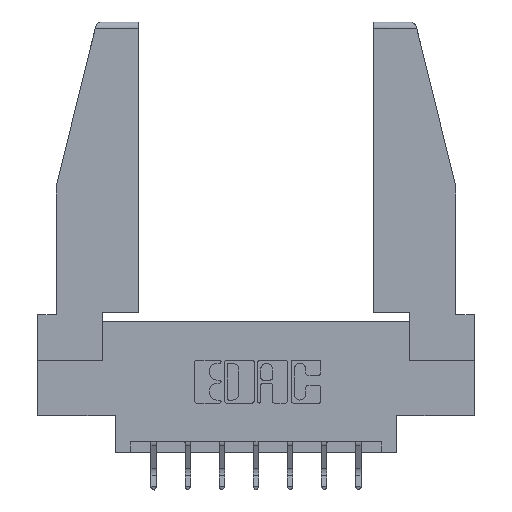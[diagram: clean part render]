
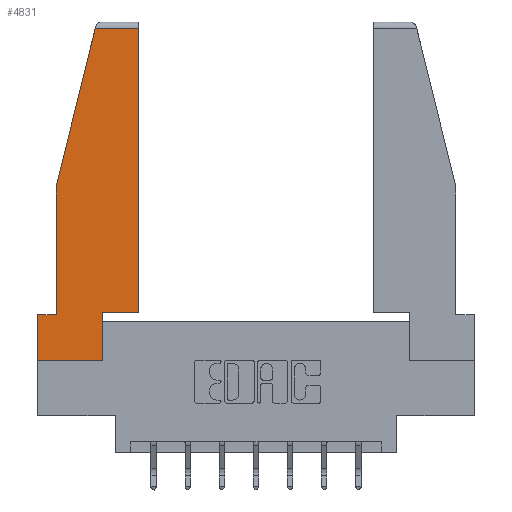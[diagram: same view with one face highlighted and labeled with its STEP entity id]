
A CAD part, top view. The second image highlights one B-rep face of the part: STEP entity #4831.
In plain terms, the highlighted planar face has unit normal (0, 0, 1).
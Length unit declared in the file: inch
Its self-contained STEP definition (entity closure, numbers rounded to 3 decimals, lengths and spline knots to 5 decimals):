
#357 = DIRECTION ( 'NONE',  ( 1., 0., 0. ) ) ;
#682 = CARTESIAN_POINT ( 'NONE',  ( 0.086, 0.21, 0. ) ) ;
#701 = CARTESIAN_POINT ( 'NONE',  ( 0.461, 1.52, 0. ) ) ;
#712 = LINE ( 'NONE', #8739, #11179 ) ;
#985 = DIRECTION ( 'NONE',  ( 1., 0., 0. ) ) ;
#1000 = DIRECTION ( 'NONE',  ( 0., 1., 0. ) ) ;
#1117 = CARTESIAN_POINT ( 'NONE',  ( 0., 1.52, 0. ) ) ;
#1374 = VECTOR ( 'NONE', #1000, 39.37008 ) ;
#1444 = ORIENTED_EDGE ( 'NONE', *, *, #9144, .T. ) ;
#1696 = EDGE_CURVE ( 'NONE', #3727, #12095, #6595, .T. ) ;
#1740 = ORIENTED_EDGE ( 'NONE', *, *, #8124, .T. ) ;
#1833 = CARTESIAN_POINT ( 'NONE',  ( 0.461, 0.223, 0. ) ) ;
#1866 = CARTESIAN_POINT ( 'NONE',  ( 0.297, 0.223, 0. ) ) ;
#1889 = CARTESIAN_POINT ( 'NONE',  ( 0.297, 0., 0. ) ) ;
#2058 = LINE ( 'NONE', #1117, #5145 ) ;
#2481 = AXIS2_PLACEMENT_3D ( 'NONE', #11705, #5888, #985 ) ;
#2533 = PLANE ( 'NONE',  #2481 ) ;
#2795 = ORIENTED_EDGE ( 'NONE', *, *, #5184, .T. ) ;
#3535 = DIRECTION ( 'NONE',  ( -0.239, -0.971, 0. ) ) ;
#3662 = ORIENTED_EDGE ( 'NONE', *, *, #4491, .T. ) ;
#3727 = VERTEX_POINT ( 'NONE', #8665 ) ;
#3953 = VECTOR ( 'NONE', #3535, 39.37008 ) ;
#4037 = CARTESIAN_POINT ( 'NONE',  ( 0., 0.21, 0. ) ) ;
#4092 = EDGE_CURVE ( 'NONE', #12095, #10787, #12732, .T. ) ;
#4183 = CARTESIAN_POINT ( 'NONE',  ( 0., 0.21, 0. ) ) ;
#4266 = DIRECTION ( 'NONE',  ( -1., 0., 0. ) ) ;
#4287 = CARTESIAN_POINT ( 'NONE',  ( 0., 0., 0. ) ) ;
#4328 = ORIENTED_EDGE ( 'NONE', *, *, #4092, .T. ) ;
#4427 = EDGE_CURVE ( 'NONE', #11639, #10561, #8569, .T. ) ;
#4432 = VECTOR ( 'NONE', #8693, 39.37008 ) ;
#4486 = EDGE_LOOP ( 'NONE', ( #9911, #5572, #12630, #4328, #1740, #2795, #1444, #11245, #3662 ) ) ;
#4491 = EDGE_CURVE ( 'NONE', #10561, #9969, #712, .T. ) ;
#4831 = ADVANCED_FACE ( 'NONE', ( #11328 ), #2533, .T. ) ;
#5145 = VECTOR ( 'NONE', #7988, 39.37008 ) ;
#5184 = EDGE_CURVE ( 'NONE', #12124, #8366, #11319, .T. ) ;
#5343 = VECTOR ( 'NONE', #10682, 39.37008 ) ;
#5572 = ORIENTED_EDGE ( 'NONE', *, *, #10342, .T. ) ;
#5845 = CARTESIAN_POINT ( 'NONE',  ( 0.086, 0.8, 0. ) ) ;
#5888 = DIRECTION ( 'NONE',  ( 0., 0., 1. ) ) ;
#6595 = LINE ( 'NONE', #11475, #3953 ) ;
#7249 = VECTOR ( 'NONE', #357, 39.37008 ) ;
#7555 = LINE ( 'NONE', #4287, #7249 ) ;
#7717 = VECTOR ( 'NONE', #4266, 39.37008 ) ;
#7988 = DIRECTION ( 'NONE',  ( -1., 0., 0. ) ) ;
#8124 = EDGE_CURVE ( 'NONE', #10787, #12124, #10316, .T. ) ;
#8366 = VERTEX_POINT ( 'NONE', #9663 ) ;
#8465 = LINE ( 'NONE', #12691, #1374 ) ;
#8569 = LINE ( 'NONE', #8664, #5343 ) ;
#8573 = EDGE_CURVE ( 'NONE', #9969, #11468, #8465, .T. ) ;
#8622 = DIRECTION ( 'NONE',  ( 1., 0., 0. ) ) ;
#8664 = CARTESIAN_POINT ( 'NONE',  ( 0.297, 0., 0. ) ) ;
#8665 = CARTESIAN_POINT ( 'NONE',  ( 0.2636, 1.52, 0. ) ) ;
#8693 = DIRECTION ( 'NONE',  ( 0., -1., 0. ) ) ;
#8739 = CARTESIAN_POINT ( 'NONE',  ( 0.297, 0.223, 0. ) ) ;
#8902 = DIRECTION ( 'NONE',  ( 0., -1., 0. ) ) ;
#9144 = EDGE_CURVE ( 'NONE', #8366, #11639, #7555, .T. ) ;
#9623 = VECTOR ( 'NONE', #8902, 39.37008 ) ;
#9663 = CARTESIAN_POINT ( 'NONE',  ( 0., 0., 0. ) ) ;
#9911 = ORIENTED_EDGE ( 'NONE', *, *, #8573, .T. ) ;
#9969 = VERTEX_POINT ( 'NONE', #1833 ) ;
#10316 = LINE ( 'NONE', #4183, #7717 ) ;
#10342 = EDGE_CURVE ( 'NONE', #11468, #3727, #2058, .T. ) ;
#10561 = VERTEX_POINT ( 'NONE', #1866 ) ;
#10682 = DIRECTION ( 'NONE',  ( 0., 1., 0. ) ) ;
#10787 = VERTEX_POINT ( 'NONE', #682 ) ;
#11179 = VECTOR ( 'NONE', #8622, 39.37008 ) ;
#11245 = ORIENTED_EDGE ( 'NONE', *, *, #4427, .T. ) ;
#11319 = LINE ( 'NONE', #4037, #9623 ) ;
#11328 = FACE_OUTER_BOUND ( 'NONE', #4486, .T. ) ;
#11468 = VERTEX_POINT ( 'NONE', #701 ) ;
#11475 = CARTESIAN_POINT ( 'NONE',  ( 0.271, 1.55, 0. ) ) ;
#11639 = VERTEX_POINT ( 'NONE', #1889 ) ;
#11677 = CARTESIAN_POINT ( 'NONE',  ( 0.086, 0.8, 0. ) ) ;
#11705 = CARTESIAN_POINT ( 'NONE',  ( 0., 0., 0. ) ) ;
#12025 = CARTESIAN_POINT ( 'NONE',  ( 0., 0.21, 0. ) ) ;
#12095 = VERTEX_POINT ( 'NONE', #5845 ) ;
#12124 = VERTEX_POINT ( 'NONE', #12025 ) ;
#12630 = ORIENTED_EDGE ( 'NONE', *, *, #1696, .T. ) ;
#12691 = CARTESIAN_POINT ( 'NONE',  ( 0.461, 0.223, 0. ) ) ;
#12732 = LINE ( 'NONE', #11677, #4432 ) ;
